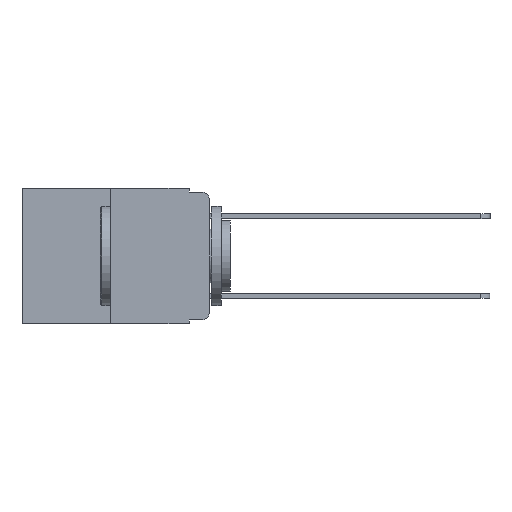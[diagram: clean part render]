
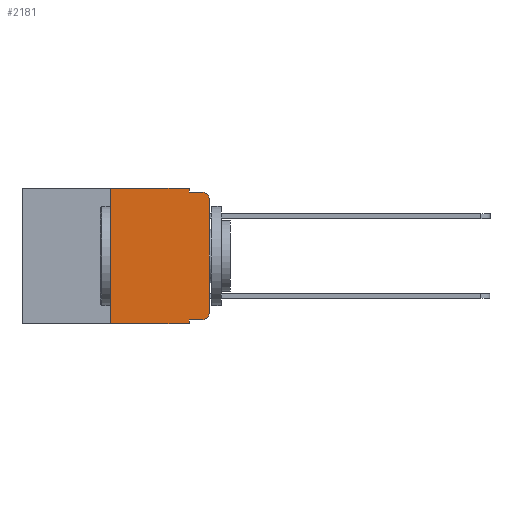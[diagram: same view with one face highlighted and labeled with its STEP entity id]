
A CAD part, left-side view. The second image highlights one B-rep face of the part: STEP entity #2181.
In plain terms, the highlighted planar face has unit normal (-1, 0, 0).
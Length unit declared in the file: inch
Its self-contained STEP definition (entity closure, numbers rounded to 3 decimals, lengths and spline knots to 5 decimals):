
#135 = LINE ( 'NONE', #2653, #4199 ) ;
#151 = CARTESIAN_POINT ( 'NONE',  ( 0., 0.051, -0.343 ) ) ;
#590 = CARTESIAN_POINT ( 'NONE',  ( 0., 0.473, 0. ) ) ;
#669 = DIRECTION ( 'NONE',  ( 0., 0., -1. ) ) ;
#684 = DIRECTION ( 'NONE',  ( 0., 0., -1. ) ) ;
#728 = DIRECTION ( 'NONE',  ( 0., -1., 0. ) ) ;
#1190 = PLANE ( 'NONE',  #7692 ) ;
#1203 = FACE_OUTER_BOUND ( 'NONE', #4447, .T. ) ;
#1236 = DIRECTION ( 'NONE',  ( 0., 0., 1. ) ) ;
#1434 = CARTESIAN_POINT ( 'NONE',  ( 0., 0.02, -0.01 ) ) ;
#1487 = DIRECTION ( 'NONE',  ( 0., 0., -1. ) ) ;
#1806 = VERTEX_POINT ( 'NONE', #8911 ) ;
#1901 = VERTEX_POINT ( 'NONE', #8460 ) ;
#2052 = LINE ( 'NONE', #4764, #4004 ) ;
#2160 = VECTOR ( 'NONE', #7706, 39.37008 ) ;
#2165 = CARTESIAN_POINT ( 'NONE',  ( 0., 0.051, -0.333 ) ) ;
#2181 = ADVANCED_FACE ( 'NONE', ( #1203 ), #1190, .F. ) ;
#2513 = DIRECTION ( 'NONE',  ( 1., 0., 0. ) ) ;
#2653 = CARTESIAN_POINT ( 'NONE',  ( 0., 0.051, 0. ) ) ;
#3004 = VERTEX_POINT ( 'NONE', #6496 ) ;
#3207 = EDGE_CURVE ( 'NONE', #7907, #8174, #6719, .T. ) ;
#3220 = CARTESIAN_POINT ( 'NONE',  ( 0., 0.473, 0. ) ) ;
#3475 = EDGE_CURVE ( 'NONE', #1901, #3004, #4377, .T. ) ;
#3566 = LINE ( 'NONE', #3875, #9583 ) ;
#3722 = EDGE_CURVE ( 'NONE', #8268, #7907, #2052, .T. ) ;
#3812 = CIRCLE ( 'NONE', #8950, 0.02 ) ;
#3875 = CARTESIAN_POINT ( 'NONE',  ( 0., 0., 0. ) ) ;
#3971 = VERTEX_POINT ( 'NONE', #1434 ) ;
#4004 = VECTOR ( 'NONE', #4778, 39.37008 ) ;
#4151 = VERTEX_POINT ( 'NONE', #151 ) ;
#4199 = VECTOR ( 'NONE', #1487, 39.37008 ) ;
#4236 = VECTOR ( 'NONE', #9022, 39.37008 ) ;
#4246 = EDGE_CURVE ( 'NONE', #8268, #4151, #10430, .T. ) ;
#4269 = DIRECTION ( 'NONE',  ( 0., -1., 0. ) ) ;
#4304 = ORIENTED_EDGE ( 'NONE', *, *, #7501, .T. ) ;
#4377 = LINE ( 'NONE', #590, #6344 ) ;
#4447 = EDGE_LOOP ( 'NONE', ( #4304, #4957, #5089, #6245, #6267, #6441, #6544, #6573, #6695, #6723 ) ) ;
#4574 = LINE ( 'NONE', #9007, #8567 ) ;
#4764 = CARTESIAN_POINT ( 'NONE',  ( 0., 0.051, -0.333 ) ) ;
#4778 = DIRECTION ( 'NONE',  ( 0., -1., 0. ) ) ;
#4806 = EDGE_CURVE ( 'NONE', #1806, #1901, #9053, .T. ) ;
#4899 = AXIS2_PLACEMENT_3D ( 'NONE', #8453, #8413, #8183 ) ;
#4928 = CARTESIAN_POINT ( 'NONE',  ( 0., 0.473, -0.343 ) ) ;
#4957 = ORIENTED_EDGE ( 'NONE', *, *, #6987, .T. ) ;
#5089 = ORIENTED_EDGE ( 'NONE', *, *, #6473, .F. ) ;
#5300 = CARTESIAN_POINT ( 'NONE',  ( 0., 0., -0.313 ) ) ;
#5352 = EDGE_CURVE ( 'NONE', #3004, #9876, #135, .T. ) ;
#5749 = CARTESIAN_POINT ( 'NONE',  ( 0., 0.051, -0.01 ) ) ;
#5777 = CARTESIAN_POINT ( 'NONE',  ( 0., 0.051, 0. ) ) ;
#5797 = DIRECTION ( 'NONE',  ( 0., -1., 0. ) ) ;
#5824 = DIRECTION ( 'NONE',  ( -1., 0., 0. ) ) ;
#6245 = ORIENTED_EDGE ( 'NONE', *, *, #5352, .F. ) ;
#6267 = ORIENTED_EDGE ( 'NONE', *, *, #3475, .F. ) ;
#6344 = VECTOR ( 'NONE', #728, 39.37008 ) ;
#6441 = ORIENTED_EDGE ( 'NONE', *, *, #4806, .F. ) ;
#6473 = EDGE_CURVE ( 'NONE', #9876, #3971, #4574, .T. ) ;
#6496 = CARTESIAN_POINT ( 'NONE',  ( 0., 0.051, 0. ) ) ;
#6544 = ORIENTED_EDGE ( 'NONE', *, *, #9343, .T. ) ;
#6573 = ORIENTED_EDGE ( 'NONE', *, *, #4246, .F. ) ;
#6695 = ORIENTED_EDGE ( 'NONE', *, *, #3722, .T. ) ;
#6719 = CIRCLE ( 'NONE', #4899, 0.02 ) ;
#6723 = ORIENTED_EDGE ( 'NONE', *, *, #3207, .T. ) ;
#6987 = EDGE_CURVE ( 'NONE', #8685, #3971, #3812, .T. ) ;
#7463 = CARTESIAN_POINT ( 'NONE',  ( 0., 0., -0.03 ) ) ;
#7501 = EDGE_CURVE ( 'NONE', #8174, #8685, #3566, .T. ) ;
#7692 = AXIS2_PLACEMENT_3D ( 'NONE', #3220, #2513, #684 ) ;
#7706 = DIRECTION ( 'NONE',  ( 0., 0., 1. ) ) ;
#7907 = VERTEX_POINT ( 'NONE', #9618 ) ;
#8174 = VERTEX_POINT ( 'NONE', #5300 ) ;
#8183 = DIRECTION ( 'NONE',  ( 0., 0., -1. ) ) ;
#8268 = VERTEX_POINT ( 'NONE', #2165 ) ;
#8413 = DIRECTION ( 'NONE',  ( -1., 0., 0. ) ) ;
#8453 = CARTESIAN_POINT ( 'NONE',  ( 0., 0.02, -0.313 ) ) ;
#8460 = CARTESIAN_POINT ( 'NONE',  ( 0., 0.25, 0. ) ) ;
#8567 = VECTOR ( 'NONE', #4269, 39.37008 ) ;
#8685 = VERTEX_POINT ( 'NONE', #7463 ) ;
#8911 = CARTESIAN_POINT ( 'NONE',  ( 0., 0.25, -0.343 ) ) ;
#8950 = AXIS2_PLACEMENT_3D ( 'NONE', #10334, #5824, #669 ) ;
#9007 = CARTESIAN_POINT ( 'NONE',  ( 0., 0.051, -0.01 ) ) ;
#9022 = DIRECTION ( 'NONE',  ( 0., 0., -1. ) ) ;
#9053 = LINE ( 'NONE', #10006, #2160 ) ;
#9343 = EDGE_CURVE ( 'NONE', #1806, #4151, #9582, .T. ) ;
#9356 = VECTOR ( 'NONE', #5797, 39.37008 ) ;
#9582 = LINE ( 'NONE', #4928, #9356 ) ;
#9583 = VECTOR ( 'NONE', #1236, 39.37008 ) ;
#9618 = CARTESIAN_POINT ( 'NONE',  ( 0., 0.02, -0.333 ) ) ;
#9876 = VERTEX_POINT ( 'NONE', #5749 ) ;
#10006 = CARTESIAN_POINT ( 'NONE',  ( 0., 0.25, 0. ) ) ;
#10334 = CARTESIAN_POINT ( 'NONE',  ( 0., 0.02, -0.03 ) ) ;
#10430 = LINE ( 'NONE', #5777, #4236 ) ;
